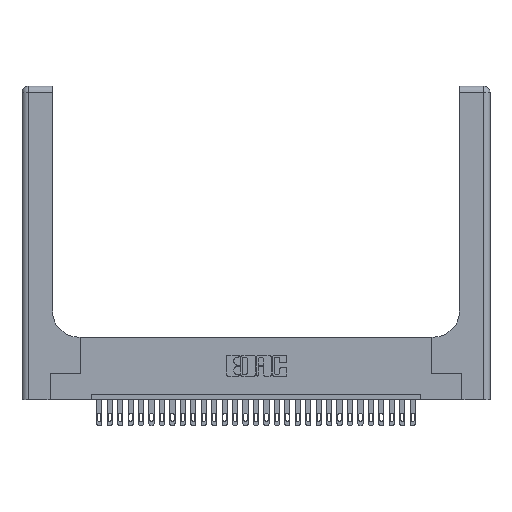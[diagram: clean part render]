
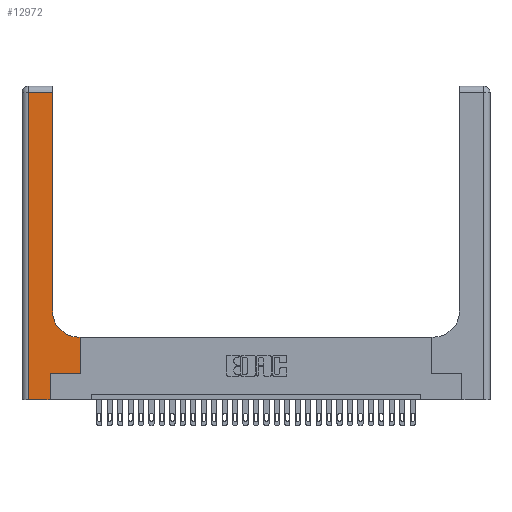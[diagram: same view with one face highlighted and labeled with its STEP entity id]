
A CAD part, top view. The second image highlights one B-rep face of the part: STEP entity #12972.
In plain terms, the highlighted planar face has unit normal (0, 0, 1).
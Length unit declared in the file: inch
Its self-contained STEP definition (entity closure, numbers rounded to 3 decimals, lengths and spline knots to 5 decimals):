
#623 = DIRECTION ( 'NONE',  ( 0., 1., 0. ) ) ;
#1222 = VERTEX_POINT ( 'NONE', #5695 ) ;
#1704 = LINE ( 'NONE', #25714, #21129 ) ;
#2084 = VERTEX_POINT ( 'NONE', #14582 ) ;
#3044 = CARTESIAN_POINT ( 'NONE',  ( 0.5585, 0.6, 0.37 ) ) ;
#3846 = CARTESIAN_POINT ( 'NONE',  ( 0.5585, 0.25, 0.37 ) ) ;
#5695 = CARTESIAN_POINT ( 'NONE',  ( 0.2915, 2.94, 0.37 ) ) ;
#6298 = CARTESIAN_POINT ( 'NONE',  ( 0.2915, 0.85, 0.37 ) ) ;
#6413 = EDGE_CURVE ( 'NONE', #2084, #9492, #17964, .T. ) ;
#7124 = CARTESIAN_POINT ( 'NONE',  ( 0., 2.94, 0.37 ) ) ;
#7264 = DIRECTION ( 'NONE',  ( 1., 0., 0. ) ) ;
#7423 = EDGE_CURVE ( 'NONE', #26511, #16460, #1704, .T. ) ;
#7775 = VERTEX_POINT ( 'NONE', #3044 ) ;
#8518 = CARTESIAN_POINT ( 'NONE',  ( 0.06, 0., 0.37 ) ) ;
#9067 = LINE ( 'NONE', #7124, #21656 ) ;
#9121 = AXIS2_PLACEMENT_3D ( 'NONE', #23887, #23684, #10311 ) ;
#9492 = VERTEX_POINT ( 'NONE', #23505 ) ;
#9978 = EDGE_CURVE ( 'NONE', #16460, #2084, #14499, .T. ) ;
#10114 = PLANE ( 'NONE',  #9121 ) ;
#10311 = DIRECTION ( 'NONE',  ( -1., 0., 0. ) ) ;
#10438 = FACE_OUTER_BOUND ( 'NONE', #13412, .T. ) ;
#10482 = VERTEX_POINT ( 'NONE', #6298 ) ;
#11822 = VECTOR ( 'NONE', #18961, 39.37008 ) ;
#12559 = DIRECTION ( 'NONE',  ( 1., 0., 0. ) ) ;
#12972 = ADVANCED_FACE ( 'NONE', ( #10438 ), #10114, .F. ) ;
#13412 = EDGE_LOOP ( 'NONE', ( #28433, #17757, #21587, #26934, #25134, #27403, #22568, #26923, #28482 ) ) ;
#13509 = CARTESIAN_POINT ( 'NONE',  ( 0.2915, 3., 0.37 ) ) ;
#14499 = LINE ( 'NONE', #15092, #29734 ) ;
#14582 = CARTESIAN_POINT ( 'NONE',  ( 0.269, 0.25, 0.37 ) ) ;
#14914 = CARTESIAN_POINT ( 'NONE',  ( 0.06, 3., 0.37 ) ) ;
#15092 = CARTESIAN_POINT ( 'NONE',  ( 0.269, 0., 0.37 ) ) ;
#15234 = AXIS2_PLACEMENT_3D ( 'NONE', #26241, #28372, #12559 ) ;
#15419 = CARTESIAN_POINT ( 'NONE',  ( 0.2915, 0.6, 0.37 ) ) ;
#15741 = CIRCLE ( 'NONE', #15234, 0.25 ) ;
#16460 = VERTEX_POINT ( 'NONE', #22537 ) ;
#17757 = ORIENTED_EDGE ( 'NONE', *, *, #19850, .T. ) ;
#17964 = LINE ( 'NONE', #28264, #11822 ) ;
#18402 = CARTESIAN_POINT ( 'NONE',  ( 0.06, 2.94, 0.37 ) ) ;
#18750 = VERTEX_POINT ( 'NONE', #22395 ) ;
#18961 = DIRECTION ( 'NONE',  ( 1., 0., 0. ) ) ;
#19411 = DIRECTION ( 'NONE',  ( 0., 1., 0. ) ) ;
#19752 = DIRECTION ( 'NONE',  ( 0., -1., 0. ) ) ;
#19770 = EDGE_CURVE ( 'NONE', #20812, #26511, #23451, .T. ) ;
#19850 = EDGE_CURVE ( 'NONE', #1222, #20812, #9067, .T. ) ;
#19989 = DIRECTION ( 'NONE',  ( 0., 1., 0. ) ) ;
#20812 = VERTEX_POINT ( 'NONE', #18402 ) ;
#21129 = VECTOR ( 'NONE', #7264, 39.37008 ) ;
#21587 = ORIENTED_EDGE ( 'NONE', *, *, #19770, .T. ) ;
#21656 = VECTOR ( 'NONE', #25256, 39.37008 ) ;
#21726 = LINE ( 'NONE', #13509, #23523 ) ;
#22395 = CARTESIAN_POINT ( 'NONE',  ( 0.5415, 0.6, 0.37 ) ) ;
#22537 = CARTESIAN_POINT ( 'NONE',  ( 0.269, 0., 0.37 ) ) ;
#22568 = ORIENTED_EDGE ( 'NONE', *, *, #22809, .T. ) ;
#22809 = EDGE_CURVE ( 'NONE', #9492, #7775, #23073, .T. ) ;
#23073 = LINE ( 'NONE', #3846, #24825 ) ;
#23451 = LINE ( 'NONE', #14914, #27069 ) ;
#23505 = CARTESIAN_POINT ( 'NONE',  ( 0.5585, 0.25, 0.37 ) ) ;
#23523 = VECTOR ( 'NONE', #623, 39.37008 ) ;
#23684 = DIRECTION ( 'NONE',  ( 0., 0., -1. ) ) ;
#23887 = CARTESIAN_POINT ( 'NONE',  ( 0., 3., 0.37 ) ) ;
#24171 = LINE ( 'NONE', #15419, #24890 ) ;
#24461 = DIRECTION ( 'NONE',  ( -1., 0., 0. ) ) ;
#24825 = VECTOR ( 'NONE', #19989, 39.37008 ) ;
#24890 = VECTOR ( 'NONE', #24461, 39.37008 ) ;
#25134 = ORIENTED_EDGE ( 'NONE', *, *, #9978, .T. ) ;
#25256 = DIRECTION ( 'NONE',  ( -1., 0., 0. ) ) ;
#25261 = EDGE_CURVE ( 'NONE', #18750, #10482, #15741, .T. ) ;
#25714 = CARTESIAN_POINT ( 'NONE',  ( 0., 0., 0.37 ) ) ;
#26241 = CARTESIAN_POINT ( 'NONE',  ( 0.5415, 0.85, 0.37 ) ) ;
#26511 = VERTEX_POINT ( 'NONE', #8518 ) ;
#26923 = ORIENTED_EDGE ( 'NONE', *, *, #28795, .T. ) ;
#26934 = ORIENTED_EDGE ( 'NONE', *, *, #7423, .T. ) ;
#27069 = VECTOR ( 'NONE', #19752, 39.37008 ) ;
#27403 = ORIENTED_EDGE ( 'NONE', *, *, #6413, .T. ) ;
#27793 = EDGE_CURVE ( 'NONE', #10482, #1222, #21726, .T. ) ;
#28264 = CARTESIAN_POINT ( 'NONE',  ( 0.269, 0.25, 0.37 ) ) ;
#28372 = DIRECTION ( 'NONE',  ( 0., 0., -1. ) ) ;
#28433 = ORIENTED_EDGE ( 'NONE', *, *, #27793, .T. ) ;
#28482 = ORIENTED_EDGE ( 'NONE', *, *, #25261, .T. ) ;
#28795 = EDGE_CURVE ( 'NONE', #7775, #18750, #24171, .T. ) ;
#29734 = VECTOR ( 'NONE', #19411, 39.37008 ) ;
